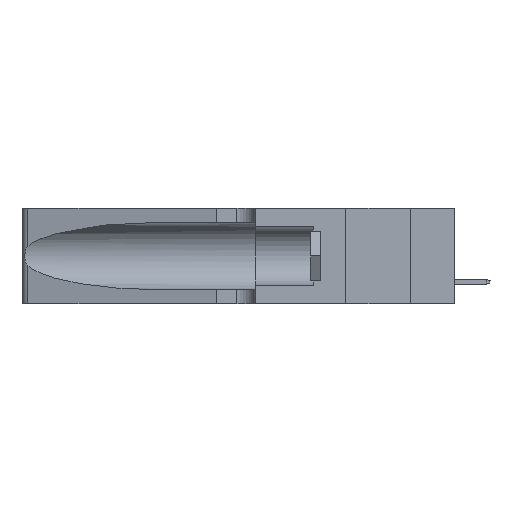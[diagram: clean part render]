
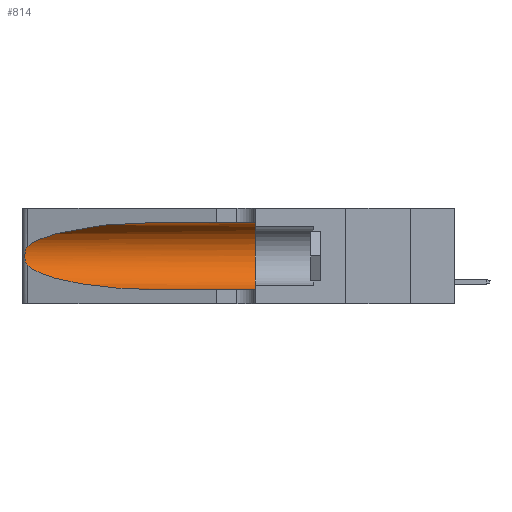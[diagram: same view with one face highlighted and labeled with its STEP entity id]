
A CAD part, left-side view. The second image highlights one B-rep face of the part: STEP entity #814.
In plain terms, the highlighted cylindrical face has radius 3.308 mm (diameter 6.617 mm), a partial arc.
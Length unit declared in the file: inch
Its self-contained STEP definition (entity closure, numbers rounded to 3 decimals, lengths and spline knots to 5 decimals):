
#814 = ADVANCED_FACE ( 'NONE', ( #19950 ), #5768, .F. ) ;
#1984 = EDGE_CURVE ( 'NONE', #15735, #6327, #37662, .T. ) ;
#2802 = CARTESIAN_POINT ( 'NONE',  ( 0.1305, 0.72297, 0.05475 ) ) ;
#3257 = LINE ( 'NONE', #17050, #34613 ) ;
#3523 = EDGE_CURVE ( 'NONE', #7139, #13337, #4218, .T. ) ;
#4121 = CARTESIAN_POINT ( 'NONE',  ( 0.25487, 1.22718, 0.14631 ) ) ;
#4218 = B_SPLINE_CURVE_WITH_KNOTS ( 'NONE', 3,
 ( #24326, #17892, #11033, #41602, #20997, #34497, #7918, #24540, #31153, #38059, #28068, #7268, #37826, #4121 ),
 .UNSPECIFIED., .F., .F.,
 ( 4, 2, 2, 2, 2, 2, 4 ),
 ( 0., 0.00027, 0.00053, 0.00107, 0.0016, 0.00187, 0.00214 ),
 .UNSPECIFIED. ) ;
#5768 = CYLINDRICAL_SURFACE ( 'NONE', #15078, 0.13025 ) ;
#5812 = VECTOR ( 'NONE', #28575, 39.37008 ) ;
#6327 = VERTEX_POINT ( 'NONE', #41019 ) ;
#6556 = CARTESIAN_POINT ( 'NONE',  ( 0.1305, 0.72297, 0.31525 ) ) ;
#6883 = DIRECTION ( 'NONE',  ( 0., 0., -1. ) ) ;
#7139 = VERTEX_POINT ( 'NONE', #33366 ) ;
#7268 = CARTESIAN_POINT ( 'NONE',  ( 0.25639, 1.23186, 0.15144 ) ) ;
#7296 = EDGE_CURVE ( 'NONE', #16376, #7139, #10926, .T. ) ;
#7918 = CARTESIAN_POINT ( 'NONE',  ( 0.26075, 1.23896, 0.19203 ) ) ;
#8415 = ORIENTED_EDGE ( 'NONE', *, *, #11344, .F. ) ;
#9072 = CARTESIAN_POINT ( 'NONE',  ( 0.18966, 0.96281, 0.05475 ) ) ;
#10211 = DIRECTION ( 'NONE',  ( 0., -1., 0. ) ) ;
#10926 =( BOUNDED_CURVE ( )  B_SPLINE_CURVE ( 3, ( #17664, #15361, #14340, #42387 ),
 .UNSPECIFIED., .F., .T. ) 
 B_SPLINE_CURVE_WITH_KNOTS ( ( 4, 4 ),
 ( 1.5708, 2.84003 ),
 .UNSPECIFIED. ) 
 CURVE ( )  GEOMETRIC_REPRESENTATION_ITEM ( )  RATIONAL_B_SPLINE_CURVE ( ( 1., 0.87, 0.87, 1. ) ) 
 REPRESENTATION_ITEM ( '' )  );
#11033 = CARTESIAN_POINT ( 'NONE',  ( 0.25639, 1.23184, 0.21858 ) ) ;
#11344 = EDGE_CURVE ( 'NONE', #16376, #15735, #3257, .T. ) ;
#12021 = DIRECTION ( 'NONE',  ( 0., 0., 1. ) ) ;
#12252 = ORIENTED_EDGE ( 'NONE', *, *, #42644, .T. ) ;
#12392 = CARTESIAN_POINT ( 'NONE',  ( 0.25487, 1.22718, 0.14631 ) ) ;
#13337 = VERTEX_POINT ( 'NONE', #34229 ) ;
#13580 = ORIENTED_EDGE ( 'NONE', *, *, #20075, .T. ) ;
#14325 = EDGE_LOOP ( 'NONE', ( #42776, #40902, #12252, #13580, #28643, #8415 ) ) ;
#14340 = CARTESIAN_POINT ( 'NONE',  ( 0.2373, 1.15595, 0.28018 ) ) ;
#15078 = AXIS2_PLACEMENT_3D ( 'NONE', #41432, #10211, #6883 ) ;
#15361 = CARTESIAN_POINT ( 'NONE',  ( 0.18966, 0.96281, 0.31525 ) ) ;
#15735 = VERTEX_POINT ( 'NONE', #22144 ) ;
#16376 = VERTEX_POINT ( 'NONE', #6556 ) ;
#17050 = CARTESIAN_POINT ( 'NONE',  ( 0.1305, 1.61858, 0.31525 ) ) ;
#17664 = CARTESIAN_POINT ( 'NONE',  ( 0.1305, 0.72297, 0.31525 ) ) ;
#17892 = CARTESIAN_POINT ( 'NONE',  ( 0.25555, 1.22994, 0.2215 ) ) ;
#19237 = AXIS2_PLACEMENT_3D ( 'NONE', #29044, #39694, #12021 ) ;
#19950 = FACE_OUTER_BOUND ( 'NONE', #14325, .T. ) ;
#20075 = EDGE_CURVE ( 'NONE', #24159, #6327, #21738, .T. ) ;
#20997 = CARTESIAN_POINT ( 'NONE',  ( 0.25854, 1.2359, 0.20912 ) ) ;
#21738 = LINE ( 'NONE', #28379, #5812 ) ;
#22144 = CARTESIAN_POINT ( 'NONE',  ( 0.1305, 0.35, 0.31525 ) ) ;
#22799 = CARTESIAN_POINT ( 'NONE',  ( 0.2373, 1.15595, 0.08982 ) ) ;
#23461 = DIRECTION ( 'NONE',  ( 0., -1., 0. ) ) ;
#24159 = VERTEX_POINT ( 'NONE', #2802 ) ;
#24326 = CARTESIAN_POINT ( 'NONE',  ( 0.25487, 1.22718, 0.22369 ) ) ;
#24540 = CARTESIAN_POINT ( 'NONE',  ( 0.26075, 1.23896, 0.178 ) ) ;
#26127 = CARTESIAN_POINT ( 'NONE',  ( 0.1305, 0.72297, 0.05475 ) ) ;
#28068 = CARTESIAN_POINT ( 'NONE',  ( 0.25789, 1.23486, 0.15765 ) ) ;
#28379 = CARTESIAN_POINT ( 'NONE',  ( 0.1305, 1.61858, 0.05475 ) ) ;
#28575 = DIRECTION ( 'NONE',  ( 0., -1., 0. ) ) ;
#28643 = ORIENTED_EDGE ( 'NONE', *, *, #1984, .F. ) ;
#29044 = CARTESIAN_POINT ( 'NONE',  ( 0.1305, 0.35, 0.185 ) ) ;
#31153 = CARTESIAN_POINT ( 'NONE',  ( 0.26017, 1.23833, 0.17102 ) ) ;
#33366 = CARTESIAN_POINT ( 'NONE',  ( 0.25487, 1.22718, 0.22369 ) ) ;
#34229 = CARTESIAN_POINT ( 'NONE',  ( 0.25487, 1.22718, 0.14631 ) ) ;
#34497 = CARTESIAN_POINT ( 'NONE',  ( 0.26018, 1.23835, 0.19895 ) ) ;
#34613 = VECTOR ( 'NONE', #23461, 39.37008 ) ;
#37662 = CIRCLE ( 'NONE', #19237, 0.13025 ) ;
#37826 = CARTESIAN_POINT ( 'NONE',  ( 0.25555, 1.22993, 0.14849 ) ) ;
#38059 = CARTESIAN_POINT ( 'NONE',  ( 0.25856, 1.23593, 0.16098 ) ) ;
#38102 =( BOUNDED_CURVE ( )  B_SPLINE_CURVE ( 3, ( #12392, #22799, #9072, #26127 ),
 .UNSPECIFIED., .F., .F. ) 
 B_SPLINE_CURVE_WITH_KNOTS ( ( 4, 4 ),
 ( 3.44316, 4.71239 ),
 .UNSPECIFIED. ) 
 CURVE ( )  GEOMETRIC_REPRESENTATION_ITEM ( )  RATIONAL_B_SPLINE_CURVE ( ( 1., 0.87, 0.87, 1. ) ) 
 REPRESENTATION_ITEM ( '' )  );
#39694 = DIRECTION ( 'NONE',  ( 0., 1., 0. ) ) ;
#40902 = ORIENTED_EDGE ( 'NONE', *, *, #3523, .T. ) ;
#41019 = CARTESIAN_POINT ( 'NONE',  ( 0.1305, 0.35, 0.05475 ) ) ;
#41432 = CARTESIAN_POINT ( 'NONE',  ( 0.1305, 1.61858, 0.185 ) ) ;
#41602 = CARTESIAN_POINT ( 'NONE',  ( 0.25787, 1.23484, 0.2124 ) ) ;
#42387 = CARTESIAN_POINT ( 'NONE',  ( 0.25487, 1.22718, 0.22369 ) ) ;
#42644 = EDGE_CURVE ( 'NONE', #13337, #24159, #38102, .T. ) ;
#42776 = ORIENTED_EDGE ( 'NONE', *, *, #7296, .T. ) ;
